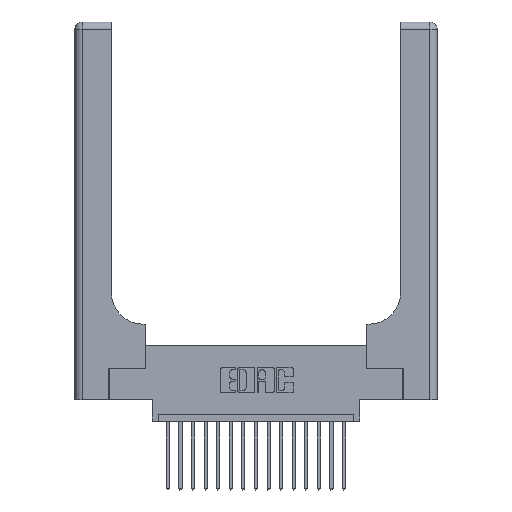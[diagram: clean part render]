
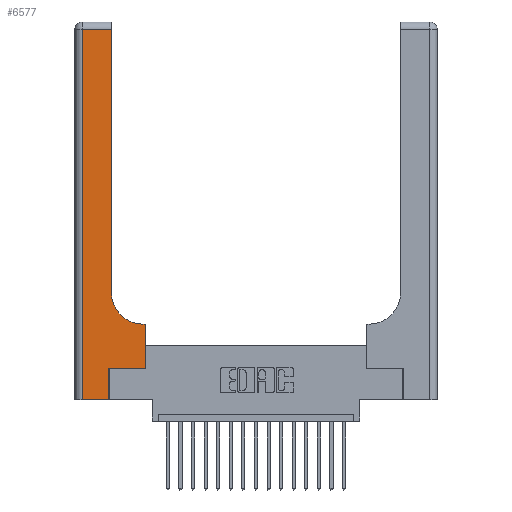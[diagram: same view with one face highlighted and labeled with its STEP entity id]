
A CAD part, top view. The second image highlights one B-rep face of the part: STEP entity #6577.
In plain terms, the highlighted planar face has unit normal (0, 0, 1).
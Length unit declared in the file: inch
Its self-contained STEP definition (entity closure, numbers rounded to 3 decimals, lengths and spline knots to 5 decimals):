
#381 = VERTEX_POINT ( 'NONE', #6326 ) ;
#681 = CARTESIAN_POINT ( 'NONE',  ( 0., 0., 0.37 ) ) ;
#885 = VECTOR ( 'NONE', #6932, 39.37008 ) ;
#1039 = ORIENTED_EDGE ( 'NONE', *, *, #11816, .T. ) ;
#1147 = LINE ( 'NONE', #17401, #15111 ) ;
#1377 = VERTEX_POINT ( 'NONE', #16772 ) ;
#1740 = EDGE_CURVE ( 'NONE', #1377, #15470, #1147, .T. ) ;
#2326 = ORIENTED_EDGE ( 'NONE', *, *, #5474, .T. ) ;
#3012 = ORIENTED_EDGE ( 'NONE', *, *, #7242, .T. ) ;
#3392 = DIRECTION ( 'NONE',  ( -1., 0., 0. ) ) ;
#3871 = AXIS2_PLACEMENT_3D ( 'NONE', #12202, #13767, #17048 ) ;
#4156 = LINE ( 'NONE', #6082, #4645 ) ;
#4207 = DIRECTION ( 'NONE',  ( 0., 1., 0. ) ) ;
#4302 = LINE ( 'NONE', #16418, #885 ) ;
#4645 = VECTOR ( 'NONE', #13987, 39.37008 ) ;
#4755 = DIRECTION ( 'NONE',  ( 0., 1., 0. ) ) ;
#5083 = VECTOR ( 'NONE', #19684, 39.37008 ) ;
#5341 = VECTOR ( 'NONE', #4755, 39.37008 ) ;
#5474 = EDGE_CURVE ( 'NONE', #6708, #15052, #20110, .T. ) ;
#6082 = CARTESIAN_POINT ( 'NONE',  ( 0.2915, 3., 0.37 ) ) ;
#6326 = CARTESIAN_POINT ( 'NONE',  ( 0.269, 0., 0.37 ) ) ;
#6436 = EDGE_CURVE ( 'NONE', #20160, #6708, #4156, .T. ) ;
#6477 = DIRECTION ( 'NONE',  ( 0., 0., -1. ) ) ;
#6577 = ADVANCED_FACE ( 'NONE', ( #17419 ), #14448, .F. ) ;
#6708 = VERTEX_POINT ( 'NONE', #11631 ) ;
#6932 = DIRECTION ( 'NONE',  ( 1., 0., 0. ) ) ;
#7242 = EDGE_CURVE ( 'NONE', #14285, #1377, #12727, .T. ) ;
#7447 = ORIENTED_EDGE ( 'NONE', *, *, #14612, .T. ) ;
#7490 = CARTESIAN_POINT ( 'NONE',  ( 0.06, 2.94, 0.37 ) ) ;
#7588 = EDGE_CURVE ( 'NONE', #15052, #19460, #17366, .T. ) ;
#7827 = CARTESIAN_POINT ( 'NONE',  ( 0.5585, 0.25, 0.37 ) ) ;
#8106 = CARTESIAN_POINT ( 'NONE',  ( 0.5585, 0.25, 0.37 ) ) ;
#8339 = DIRECTION ( 'NONE',  ( 1., 0., 0. ) ) ;
#8698 = CARTESIAN_POINT ( 'NONE',  ( 0.06, 3., 0.37 ) ) ;
#8869 = LINE ( 'NONE', #681, #17501 ) ;
#8934 = ORIENTED_EDGE ( 'NONE', *, *, #1740, .T. ) ;
#9105 = CARTESIAN_POINT ( 'NONE',  ( 0.269, 0., 0.37 ) ) ;
#9155 = VERTEX_POINT ( 'NONE', #15333 ) ;
#9744 = EDGE_CURVE ( 'NONE', #9155, #14285, #4302, .T. ) ;
#11119 = EDGE_LOOP ( 'NONE', ( #16512, #2326, #13841, #13739, #7447, #14609, #3012, #8934, #1039 ) ) ;
#11480 = CARTESIAN_POINT ( 'NONE',  ( 0., 2.94, 0.37 ) ) ;
#11631 = CARTESIAN_POINT ( 'NONE',  ( 0.2915, 2.94, 0.37 ) ) ;
#11816 = EDGE_CURVE ( 'NONE', #15470, #20160, #12811, .T. ) ;
#12130 = CARTESIAN_POINT ( 'NONE',  ( 0.2915, 0.85, 0.37 ) ) ;
#12202 = CARTESIAN_POINT ( 'NONE',  ( 0.5415, 0.85, 0.37 ) ) ;
#12727 = LINE ( 'NONE', #7827, #5341 ) ;
#12811 = CIRCLE ( 'NONE', #3871, 0.25 ) ;
#13079 = DIRECTION ( 'NONE',  ( -1., 0., 0. ) ) ;
#13739 = ORIENTED_EDGE ( 'NONE', *, *, #15190, .T. ) ;
#13767 = DIRECTION ( 'NONE',  ( 0., 0., -1. ) ) ;
#13841 = ORIENTED_EDGE ( 'NONE', *, *, #7588, .T. ) ;
#13984 = VECTOR ( 'NONE', #13079, 39.37008 ) ;
#13987 = DIRECTION ( 'NONE',  ( 0., 1., 0. ) ) ;
#14060 = AXIS2_PLACEMENT_3D ( 'NONE', #17619, #6477, #3392 ) ;
#14285 = VERTEX_POINT ( 'NONE', #8106 ) ;
#14448 = PLANE ( 'NONE',  #14060 ) ;
#14609 = ORIENTED_EDGE ( 'NONE', *, *, #9744, .T. ) ;
#14612 = EDGE_CURVE ( 'NONE', #381, #9155, #18752, .T. ) ;
#15052 = VERTEX_POINT ( 'NONE', #7490 ) ;
#15111 = VECTOR ( 'NONE', #15543, 39.37008 ) ;
#15190 = EDGE_CURVE ( 'NONE', #19460, #381, #8869, .T. ) ;
#15333 = CARTESIAN_POINT ( 'NONE',  ( 0.269, 0.25, 0.37 ) ) ;
#15470 = VERTEX_POINT ( 'NONE', #17626 ) ;
#15543 = DIRECTION ( 'NONE',  ( -1., 0., 0. ) ) ;
#16418 = CARTESIAN_POINT ( 'NONE',  ( 0.269, 0.25, 0.37 ) ) ;
#16512 = ORIENTED_EDGE ( 'NONE', *, *, #6436, .T. ) ;
#16550 = VECTOR ( 'NONE', #4207, 39.37008 ) ;
#16600 = CARTESIAN_POINT ( 'NONE',  ( 0.06, 0., 0.37 ) ) ;
#16772 = CARTESIAN_POINT ( 'NONE',  ( 0.5585, 0.6, 0.37 ) ) ;
#17048 = DIRECTION ( 'NONE',  ( 1., 0., 0. ) ) ;
#17366 = LINE ( 'NONE', #8698, #5083 ) ;
#17401 = CARTESIAN_POINT ( 'NONE',  ( 0.2915, 0.6, 0.37 ) ) ;
#17419 = FACE_OUTER_BOUND ( 'NONE', #11119, .T. ) ;
#17501 = VECTOR ( 'NONE', #8339, 39.37008 ) ;
#17619 = CARTESIAN_POINT ( 'NONE',  ( 0., 3., 0.37 ) ) ;
#17626 = CARTESIAN_POINT ( 'NONE',  ( 0.5415, 0.6, 0.37 ) ) ;
#18752 = LINE ( 'NONE', #9105, #16550 ) ;
#19460 = VERTEX_POINT ( 'NONE', #16600 ) ;
#19684 = DIRECTION ( 'NONE',  ( 0., -1., 0. ) ) ;
#20110 = LINE ( 'NONE', #11480, #13984 ) ;
#20160 = VERTEX_POINT ( 'NONE', #12130 ) ;
